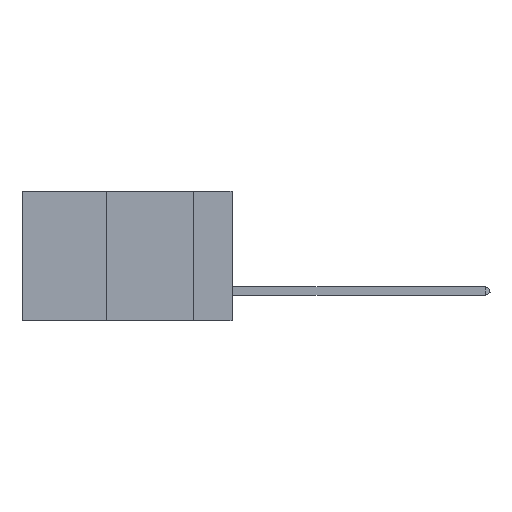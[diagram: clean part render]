
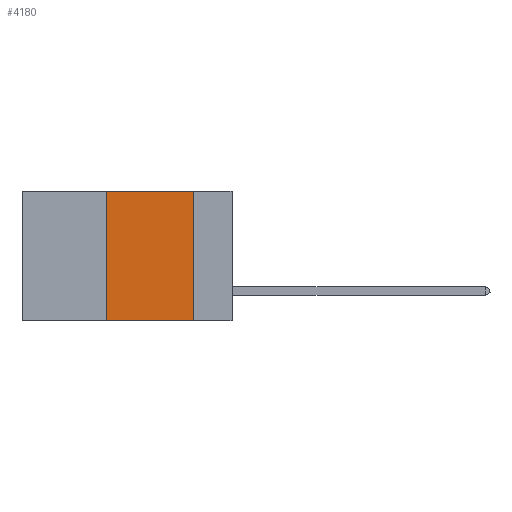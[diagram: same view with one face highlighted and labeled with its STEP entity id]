
A CAD part, left-side view. The second image highlights one B-rep face of the part: STEP entity #4180.
In plain terms, the highlighted planar face has unit normal (-1, 0, 0).
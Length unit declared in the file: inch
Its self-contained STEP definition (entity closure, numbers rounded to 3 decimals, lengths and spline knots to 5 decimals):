
#147 = LINE ( 'NONE', #267, #7963 ) ;
#218 = DIRECTION ( 'NONE',  ( 0., -1., 0. ) ) ;
#267 = CARTESIAN_POINT ( 'NONE',  ( 0., 0.6, 0. ) ) ;
#634 = ORIENTED_EDGE ( 'NONE', *, *, #5760, .F. ) ;
#805 = DIRECTION ( 'NONE',  ( 0., 0., -1. ) ) ;
#857 = VECTOR ( 'NONE', #10480, 39.37008 ) ;
#2628 = CARTESIAN_POINT ( 'NONE',  ( 0., 0.36, 0. ) ) ;
#2806 = DIRECTION ( 'NONE',  ( 0., 0., 1. ) ) ;
#3436 = ORIENTED_EDGE ( 'NONE', *, *, #5958, .F. ) ;
#3468 = DIRECTION ( 'NONE',  ( 0., 0., -1. ) ) ;
#3943 = EDGE_CURVE ( 'NONE', #10077, #12505, #10604, .T. ) ;
#4180 = ADVANCED_FACE ( 'NONE', ( #12800 ), #11175, .F. ) ;
#4781 = LINE ( 'NONE', #10562, #12420 ) ;
#5071 = CARTESIAN_POINT ( 'NONE',  ( 0., 0.6, 0. ) ) ;
#5151 = CARTESIAN_POINT ( 'NONE',  ( 0., 0.36, 0. ) ) ;
#5347 = VERTEX_POINT ( 'NONE', #12261 ) ;
#5760 = EDGE_CURVE ( 'NONE', #5347, #12505, #4781, .T. ) ;
#5958 = EDGE_CURVE ( 'NONE', #10077, #7387, #13060, .T. ) ;
#6339 = EDGE_LOOP ( 'NONE', ( #634, #6813, #3436, #7540 ) ) ;
#6561 = CARTESIAN_POINT ( 'NONE',  ( 0., 0.6, -0.37 ) ) ;
#6813 = ORIENTED_EDGE ( 'NONE', *, *, #6868, .F. ) ;
#6868 = EDGE_CURVE ( 'NONE', #7387, #5347, #147, .T. ) ;
#7387 = VERTEX_POINT ( 'NONE', #5151 ) ;
#7540 = ORIENTED_EDGE ( 'NONE', *, *, #3943, .T. ) ;
#7788 = AXIS2_PLACEMENT_3D ( 'NONE', #5071, #12186, #805 ) ;
#7963 = VECTOR ( 'NONE', #218, 39.37008 ) ;
#8160 = CARTESIAN_POINT ( 'NONE',  ( 0., 0.36, -0.37 ) ) ;
#10073 = VECTOR ( 'NONE', #2806, 39.37008 ) ;
#10077 = VERTEX_POINT ( 'NONE', #8160 ) ;
#10480 = DIRECTION ( 'NONE',  ( 0., -1., 0. ) ) ;
#10562 = CARTESIAN_POINT ( 'NONE',  ( 0., 0.11, 0. ) ) ;
#10604 = LINE ( 'NONE', #6561, #857 ) ;
#11175 = PLANE ( 'NONE',  #7788 ) ;
#12186 = DIRECTION ( 'NONE',  ( 1., 0., 0. ) ) ;
#12261 = CARTESIAN_POINT ( 'NONE',  ( 0., 0.11, 0. ) ) ;
#12420 = VECTOR ( 'NONE', #3468, 39.37008 ) ;
#12505 = VERTEX_POINT ( 'NONE', #12828 ) ;
#12800 = FACE_OUTER_BOUND ( 'NONE', #6339, .T. ) ;
#12828 = CARTESIAN_POINT ( 'NONE',  ( 0., 0.11, -0.37 ) ) ;
#13060 = LINE ( 'NONE', #2628, #10073 ) ;
